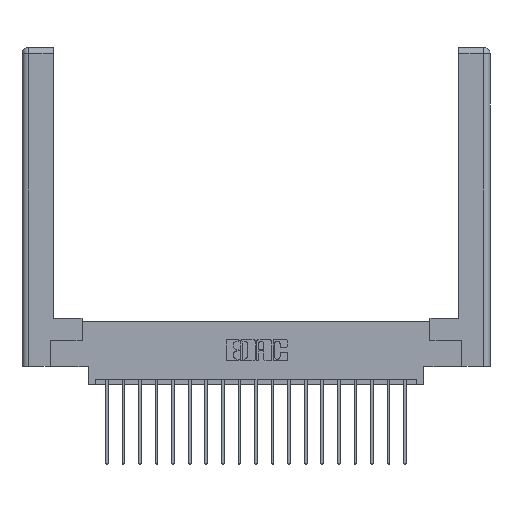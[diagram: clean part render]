
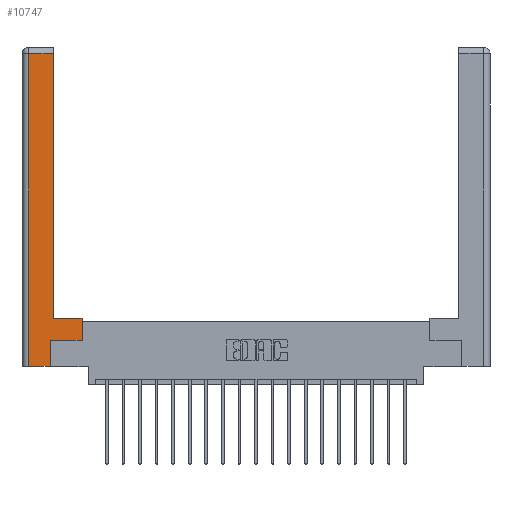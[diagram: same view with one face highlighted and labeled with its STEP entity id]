
A CAD part, top view. The second image highlights one B-rep face of the part: STEP entity #10747.
In plain terms, the highlighted planar face has unit normal (0, 0, 1).
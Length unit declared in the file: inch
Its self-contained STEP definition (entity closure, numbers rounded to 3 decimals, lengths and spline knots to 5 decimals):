
#16 = CARTESIAN_POINT ( 'NONE',  ( 0.295, 0.45, 0. ) ) ;
#89 = ORIENTED_EDGE ( 'NONE', *, *, #11336, .T. ) ;
#145 = VERTEX_POINT ( 'NONE', #13394 ) ;
#263 = EDGE_CURVE ( 'NONE', #20302, #7839, #7652, .T. ) ;
#341 = CARTESIAN_POINT ( 'NONE',  ( 0.0615, 2.94, 0. ) ) ;
#864 = CARTESIAN_POINT ( 'NONE',  ( 0.295, 0.45, 0. ) ) ;
#2205 = VERTEX_POINT ( 'NONE', #9782 ) ;
#2635 = ORIENTED_EDGE ( 'NONE', *, *, #15552, .T. ) ;
#2785 = CARTESIAN_POINT ( 'NONE',  ( 0.565, 0.245, 0. ) ) ;
#2884 = CARTESIAN_POINT ( 'NONE',  ( 0.565, 0.45, 0. ) ) ;
#3016 = ORIENTED_EDGE ( 'NONE', *, *, #5507, .T. ) ;
#3414 = VECTOR ( 'NONE', #17949, 39.37008 ) ;
#3617 = CARTESIAN_POINT ( 'NONE',  ( 0.265, 0.245, 0. ) ) ;
#3695 = VERTEX_POINT ( 'NONE', #15020 ) ;
#4041 = PLANE ( 'NONE',  #5280 ) ;
#4108 = DIRECTION ( 'NONE',  ( 0., 0., -1. ) ) ;
#4113 = CARTESIAN_POINT ( 'NONE',  ( 0.0615, 2.94, 0. ) ) ;
#4277 = LINE ( 'NONE', #2785, #12203 ) ;
#4635 = VECTOR ( 'NONE', #14102, 39.37008 ) ;
#5280 = AXIS2_PLACEMENT_3D ( 'NONE', #18273, #4108, #19886 ) ;
#5507 = EDGE_CURVE ( 'NONE', #17639, #3695, #16548, .T. ) ;
#5757 = DIRECTION ( 'NONE',  ( -1., 0., 0. ) ) ;
#6173 = VECTOR ( 'NONE', #18624, 39.37008 ) ;
#6200 = EDGE_LOOP ( 'NONE', ( #3016, #13178, #15921, #18352, #6943, #12029, #2635, #89 ) ) ;
#6559 = CARTESIAN_POINT ( 'NONE',  ( 0.565, 0.45, 0. ) ) ;
#6943 = ORIENTED_EDGE ( 'NONE', *, *, #16220, .T. ) ;
#7227 = DIRECTION ( 'NONE',  ( -1., 0., 0. ) ) ;
#7652 = LINE ( 'NONE', #8930, #16002 ) ;
#7839 = VERTEX_POINT ( 'NONE', #17670 ) ;
#8027 = LINE ( 'NONE', #864, #13701 ) ;
#8235 = EDGE_CURVE ( 'NONE', #7839, #2205, #13311, .T. ) ;
#8930 = CARTESIAN_POINT ( 'NONE',  ( 0.0615, 0., 0. ) ) ;
#9314 = VECTOR ( 'NONE', #18831, 39.37008 ) ;
#9626 = CARTESIAN_POINT ( 'NONE',  ( 0.295, 3., 0. ) ) ;
#9782 = CARTESIAN_POINT ( 'NONE',  ( 0.265, 0., 0. ) ) ;
#10747 = ADVANCED_FACE ( 'NONE', ( #11997 ), #4041, .F. ) ;
#11336 = EDGE_CURVE ( 'NONE', #20209, #17639, #8027, .T. ) ;
#11997 = FACE_OUTER_BOUND ( 'NONE', #6200, .T. ) ;
#12029 = ORIENTED_EDGE ( 'NONE', *, *, #18025, .T. ) ;
#12056 = EDGE_CURVE ( 'NONE', #3695, #20302, #12927, .T. ) ;
#12203 = VECTOR ( 'NONE', #13801, 39.37008 ) ;
#12330 = VERTEX_POINT ( 'NONE', #3617 ) ;
#12498 = CARTESIAN_POINT ( 'NONE',  ( 0.265, 0., 0. ) ) ;
#12927 = LINE ( 'NONE', #4113, #16135 ) ;
#13178 = ORIENTED_EDGE ( 'NONE', *, *, #12056, .T. ) ;
#13311 = LINE ( 'NONE', #12498, #6173 ) ;
#13394 = CARTESIAN_POINT ( 'NONE',  ( 0.565, 0.245, 0. ) ) ;
#13501 = LINE ( 'NONE', #15720, #9314 ) ;
#13701 = VECTOR ( 'NONE', #7227, 39.37008 ) ;
#13801 = DIRECTION ( 'NONE',  ( 1., 0., 0. ) ) ;
#14102 = DIRECTION ( 'NONE',  ( 0., 1., 0. ) ) ;
#15020 = CARTESIAN_POINT ( 'NONE',  ( 0.295, 2.94, 0. ) ) ;
#15552 = EDGE_CURVE ( 'NONE', #145, #20209, #17964, .T. ) ;
#15720 = CARTESIAN_POINT ( 'NONE',  ( 0.265, 0.245, 0. ) ) ;
#15921 = ORIENTED_EDGE ( 'NONE', *, *, #263, .T. ) ;
#16002 = VECTOR ( 'NONE', #16646, 39.37008 ) ;
#16135 = VECTOR ( 'NONE', #5757, 39.37008 ) ;
#16220 = EDGE_CURVE ( 'NONE', #2205, #12330, #13501, .T. ) ;
#16548 = LINE ( 'NONE', #9626, #3414 ) ;
#16646 = DIRECTION ( 'NONE',  ( 0., -1., 0. ) ) ;
#17639 = VERTEX_POINT ( 'NONE', #16 ) ;
#17670 = CARTESIAN_POINT ( 'NONE',  ( 0.0615, 0., 0. ) ) ;
#17949 = DIRECTION ( 'NONE',  ( 0., 1., 0. ) ) ;
#17964 = LINE ( 'NONE', #2884, #4635 ) ;
#18025 = EDGE_CURVE ( 'NONE', #12330, #145, #4277, .T. ) ;
#18273 = CARTESIAN_POINT ( 'NONE',  ( 0., 0., 0. ) ) ;
#18352 = ORIENTED_EDGE ( 'NONE', *, *, #8235, .T. ) ;
#18624 = DIRECTION ( 'NONE',  ( 1., 0., 0. ) ) ;
#18831 = DIRECTION ( 'NONE',  ( 0., 1., 0. ) ) ;
#19886 = DIRECTION ( 'NONE',  ( -1., 0., 0. ) ) ;
#20209 = VERTEX_POINT ( 'NONE', #6559 ) ;
#20302 = VERTEX_POINT ( 'NONE', #341 ) ;
